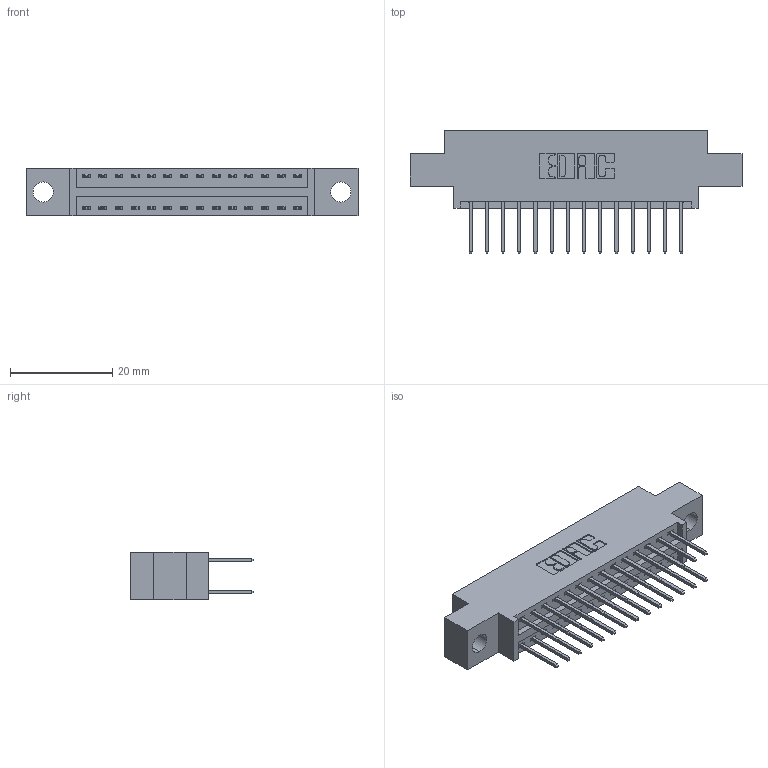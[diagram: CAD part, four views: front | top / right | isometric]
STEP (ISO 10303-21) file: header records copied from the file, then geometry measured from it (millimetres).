
FILE_DESCRIPTION (( 'STEP AP203' ), '1' );
FILE_NAME ('346-028-526-804.STEP', '2022-05-19T04:18:14', ( '' ), ( '' ), 'SwSTEP 2.0', 'SolidWorks 2020', '' );
FILE_SCHEMA (( 'CONFIG_CONTROL_DESIGN' ));
Length unit declared in the file: inch
Products named in the file (3): 346 Part_0.170 Offset - 0.156 Dia-TH; 345-292-001_345-293-126; 346-028-526-804
Assembly tree (29 placements, depth 2):
  346-028-526-804
    346 Part_0.170 Offset - 0.156 Dia-TH
    345-292-001_345-293-126  x28
Bounding box: 65.02 x 24.13 x 9.4 mm (x, y, z)
Volume: 5908.5 mm3; surface area: 7914.6 mm2
Topology: 29 solids, 29 shells, 1596 faces, 4717 edges, 3106 vertices
Faces by surface type: plane 1074, cylinder 522
Entity records: 13475 total; most frequent: CARTESIAN_POINT 2266, ORIENTED_EDGE 2198, DIRECTION 2047, EDGE_CURVE 1099, LINE 911, VECTOR 911, VERTEX_POINT 730, AXIS2_PLACEMENT_3D 568
